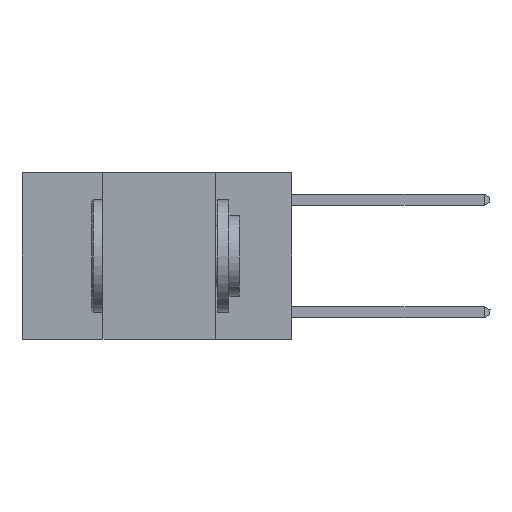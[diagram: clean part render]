
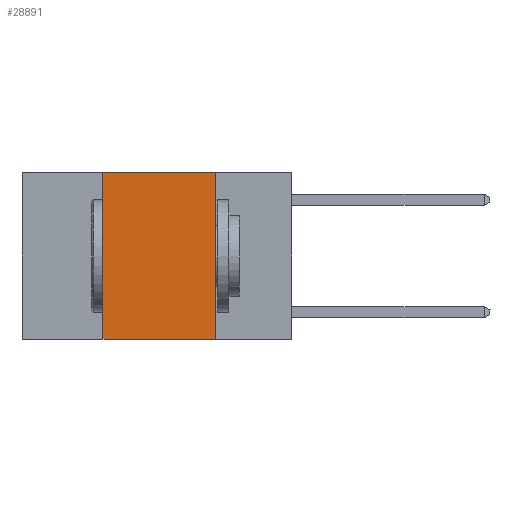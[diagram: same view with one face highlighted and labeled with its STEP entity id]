
A CAD part, left-side view. The second image highlights one B-rep face of the part: STEP entity #28891.
In plain terms, the highlighted planar face has unit normal (-1, 0, 0).
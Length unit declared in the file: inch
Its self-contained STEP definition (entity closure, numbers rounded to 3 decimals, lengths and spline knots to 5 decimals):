
#205 = EDGE_CURVE ( 'NONE', #14416, #24134, #12417, .T. ) ;
#966 = CARTESIAN_POINT ( 'NONE',  ( 0., 0.42, -0.37 ) ) ;
#1161 = LINE ( 'NONE', #28842, #5378 ) ;
#1965 = ORIENTED_EDGE ( 'NONE', *, *, #29535, .F. ) ;
#1999 = VERTEX_POINT ( 'NONE', #12038 ) ;
#5378 = VECTOR ( 'NONE', #12745, 39.37008 ) ;
#5739 = VECTOR ( 'NONE', #12064, 39.37008 ) ;
#6143 = VERTEX_POINT ( 'NONE', #20484 ) ;
#6298 = VECTOR ( 'NONE', #27383, 39.37008 ) ;
#6301 = LINE ( 'NONE', #12253, #17834 ) ;
#9786 = CARTESIAN_POINT ( 'NONE',  ( 0., 0.6, 0. ) ) ;
#10775 = ORIENTED_EDGE ( 'NONE', *, *, #19033, .T. ) ;
#11014 = EDGE_CURVE ( 'NONE', #24134, #1999, #23351, .T. ) ;
#12038 = CARTESIAN_POINT ( 'NONE',  ( 0., 0.17, 0. ) ) ;
#12064 = DIRECTION ( 'NONE',  ( 0., -1., 0. ) ) ;
#12089 = DIRECTION ( 'NONE',  ( 0., 0., -1. ) ) ;
#12253 = CARTESIAN_POINT ( 'NONE',  ( 0., 0.17, 0. ) ) ;
#12417 = LINE ( 'NONE', #22425, #6298 ) ;
#12745 = DIRECTION ( 'NONE',  ( 0., -1., 0. ) ) ;
#14416 = VERTEX_POINT ( 'NONE', #966 ) ;
#14619 = DIRECTION ( 'NONE',  ( 0., 0., -1. ) ) ;
#16717 = CARTESIAN_POINT ( 'NONE',  ( 0., 0.6, 0. ) ) ;
#17566 = AXIS2_PLACEMENT_3D ( 'NONE', #9786, #25858, #12089 ) ;
#17834 = VECTOR ( 'NONE', #14619, 39.37008 ) ;
#19033 = EDGE_CURVE ( 'NONE', #14416, #6143, #1161, .T. ) ;
#20484 = CARTESIAN_POINT ( 'NONE',  ( 0., 0.17, -0.37 ) ) ;
#21275 = EDGE_LOOP ( 'NONE', ( #1965, #29124, #21861, #10775 ) ) ;
#21636 = CARTESIAN_POINT ( 'NONE',  ( 0., 0.42, 0. ) ) ;
#21861 = ORIENTED_EDGE ( 'NONE', *, *, #205, .F. ) ;
#22425 = CARTESIAN_POINT ( 'NONE',  ( 0., 0.42, 0. ) ) ;
#23351 = LINE ( 'NONE', #16717, #5739 ) ;
#23522 = PLANE ( 'NONE',  #17566 ) ;
#24134 = VERTEX_POINT ( 'NONE', #21636 ) ;
#25858 = DIRECTION ( 'NONE',  ( 1., 0., 0. ) ) ;
#27383 = DIRECTION ( 'NONE',  ( 0., 0., 1. ) ) ;
#28842 = CARTESIAN_POINT ( 'NONE',  ( 0., 0.6, -0.37 ) ) ;
#28891 = ADVANCED_FACE ( 'NONE', ( #29046 ), #23522, .F. ) ;
#29046 = FACE_OUTER_BOUND ( 'NONE', #21275, .T. ) ;
#29124 = ORIENTED_EDGE ( 'NONE', *, *, #11014, .F. ) ;
#29535 = EDGE_CURVE ( 'NONE', #1999, #6143, #6301, .T. ) ;
